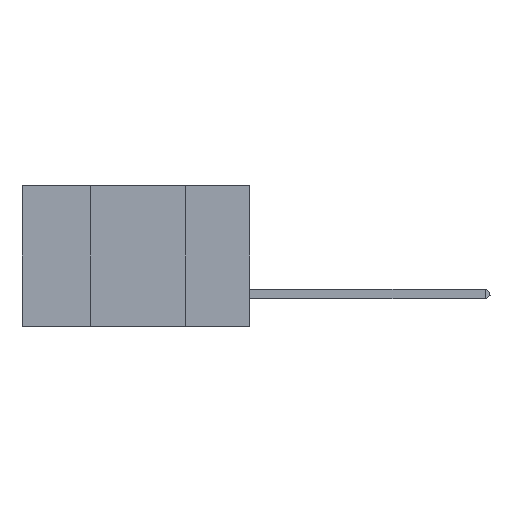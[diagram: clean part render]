
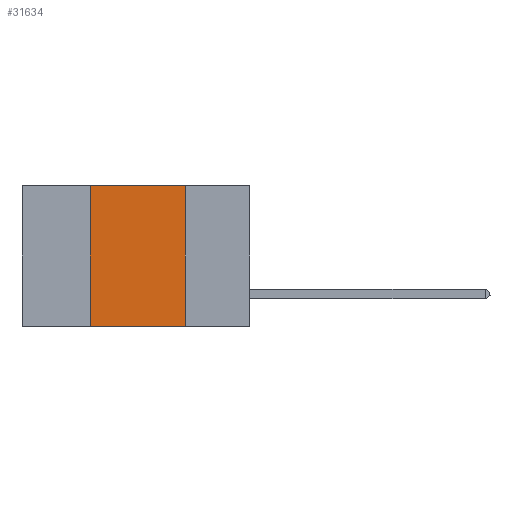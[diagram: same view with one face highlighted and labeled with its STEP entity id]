
A CAD part, left-side view. The second image highlights one B-rep face of the part: STEP entity #31634.
In plain terms, the highlighted planar face has unit normal (-1, 0, 0).
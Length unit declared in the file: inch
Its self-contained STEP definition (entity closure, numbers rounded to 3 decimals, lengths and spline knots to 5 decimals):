
#235 = LINE ( 'NONE', #40907, #4921 ) ;
#1550 = ORIENTED_EDGE ( 'NONE', *, *, #39257, .F. ) ;
#2790 = VERTEX_POINT ( 'NONE', #9579 ) ;
#4921 = VECTOR ( 'NONE', #44678, 39.37008 ) ;
#4995 = DIRECTION ( 'NONE',  ( 0., -1., 0. ) ) ;
#5584 = CARTESIAN_POINT ( 'NONE',  ( 0., 0.6, 0. ) ) ;
#7056 = VERTEX_POINT ( 'NONE', #44085 ) ;
#7692 = LINE ( 'NONE', #15836, #8896 ) ;
#8896 = VECTOR ( 'NONE', #4995, 39.37008 ) ;
#9467 = EDGE_CURVE ( 'NONE', #2790, #15106, #235, .T. ) ;
#9579 = CARTESIAN_POINT ( 'NONE',  ( 0., 0.42, -0.37 ) ) ;
#10481 = LINE ( 'NONE', #17819, #36138 ) ;
#10953 = CARTESIAN_POINT ( 'NONE',  ( 0., 0.42, 0. ) ) ;
#11409 = LINE ( 'NONE', #10953, #26510 ) ;
#14272 = ORIENTED_EDGE ( 'NONE', *, *, #42453, .F. ) ;
#15106 = VERTEX_POINT ( 'NONE', #40309 ) ;
#15836 = CARTESIAN_POINT ( 'NONE',  ( 0., 0.6, 0. ) ) ;
#17262 = DIRECTION ( 'NONE',  ( 1., 0., 0. ) ) ;
#17819 = CARTESIAN_POINT ( 'NONE',  ( 0., 0.17, 0. ) ) ;
#19204 = CARTESIAN_POINT ( 'NONE',  ( 0., 0.42, 0. ) ) ;
#19379 = FACE_OUTER_BOUND ( 'NONE', #27665, .T. ) ;
#26510 = VECTOR ( 'NONE', #33100, 39.37008 ) ;
#27128 = ORIENTED_EDGE ( 'NONE', *, *, #9467, .T. ) ;
#27665 = EDGE_LOOP ( 'NONE', ( #14272, #46653, #1550, #27128 ) ) ;
#31634 = ADVANCED_FACE ( 'NONE', ( #19379 ), #46597, .F. ) ;
#31911 = DIRECTION ( 'NONE',  ( 0., 0., -1. ) ) ;
#33100 = DIRECTION ( 'NONE',  ( 0., 0., 1. ) ) ;
#34252 = VERTEX_POINT ( 'NONE', #19204 ) ;
#36138 = VECTOR ( 'NONE', #31911, 39.37008 ) ;
#39257 = EDGE_CURVE ( 'NONE', #2790, #34252, #11409, .T. ) ;
#40309 = CARTESIAN_POINT ( 'NONE',  ( 0., 0.17, -0.37 ) ) ;
#40907 = CARTESIAN_POINT ( 'NONE',  ( 0., 0.6, -0.37 ) ) ;
#41113 = EDGE_CURVE ( 'NONE', #34252, #7056, #7692, .T. ) ;
#41951 = AXIS2_PLACEMENT_3D ( 'NONE', #5584, #17262, #47075 ) ;
#42453 = EDGE_CURVE ( 'NONE', #7056, #15106, #10481, .T. ) ;
#44085 = CARTESIAN_POINT ( 'NONE',  ( 0., 0.17, 0. ) ) ;
#44678 = DIRECTION ( 'NONE',  ( 0., -1., 0. ) ) ;
#46597 = PLANE ( 'NONE',  #41951 ) ;
#46653 = ORIENTED_EDGE ( 'NONE', *, *, #41113, .F. ) ;
#47075 = DIRECTION ( 'NONE',  ( 0., 0., -1. ) ) ;
